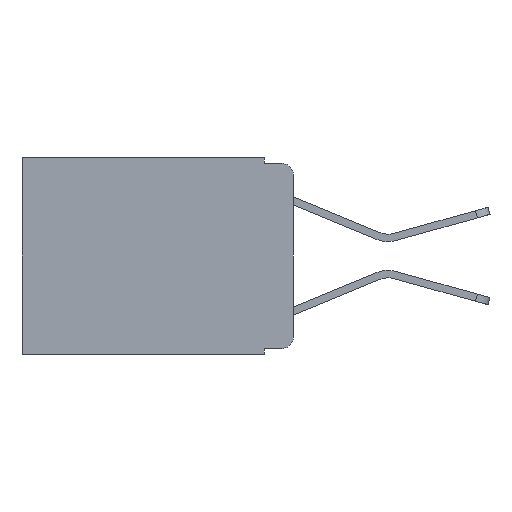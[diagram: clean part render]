
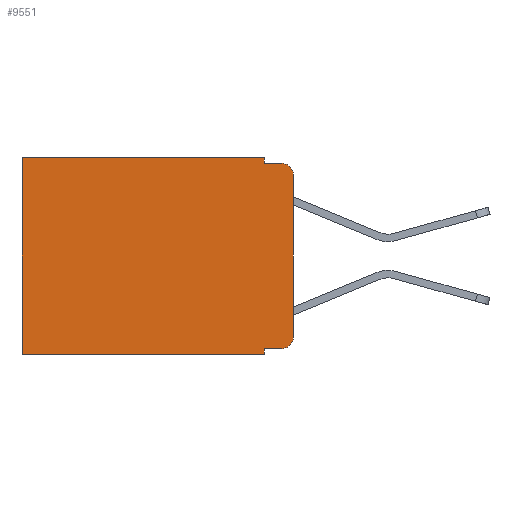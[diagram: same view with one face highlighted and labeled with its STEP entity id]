
A CAD part, left-side view. The second image highlights one B-rep face of the part: STEP entity #9551.
In plain terms, the highlighted planar face has unit normal (-1, 0, 0).
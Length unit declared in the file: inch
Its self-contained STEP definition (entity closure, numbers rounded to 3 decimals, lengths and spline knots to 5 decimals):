
#35 = ORIENTED_EDGE ( 'NONE', *, *, #2153, .T. ) ;
#64 = VERTEX_POINT ( 'NONE', #6441 ) ;
#159 = DIRECTION ( 'NONE',  ( 1., 0., 0. ) ) ;
#542 = ORIENTED_EDGE ( 'NONE', *, *, #681, .F. ) ;
#681 = EDGE_CURVE ( 'NONE', #5882, #8340, #4499, .T. ) ;
#957 = LINE ( 'NONE', #4691, #6111 ) ;
#1182 = ORIENTED_EDGE ( 'NONE', *, *, #2798, .F. ) ;
#1262 = PLANE ( 'NONE',  #4870 ) ;
#1635 = VERTEX_POINT ( 'NONE', #9061 ) ;
#1776 = CARTESIAN_POINT ( 'NONE',  ( 0.298, 0.02, -0.333 ) ) ;
#1806 = VERTEX_POINT ( 'NONE', #1776 ) ;
#2031 = EDGE_CURVE ( 'NONE', #7114, #64, #3265, .T. ) ;
#2047 = CARTESIAN_POINT ( 'NONE',  ( 0.298, 0., 0. ) ) ;
#2103 = ORIENTED_EDGE ( 'NONE', *, *, #3452, .F. ) ;
#2153 = EDGE_CURVE ( 'NONE', #5882, #10709, #8374, .T. ) ;
#2289 = CARTESIAN_POINT ( 'NONE',  ( 0.298, 0.051, -0.01 ) ) ;
#2487 = DIRECTION ( 'NONE',  ( 0., 0., -1. ) ) ;
#2606 = VECTOR ( 'NONE', #7270, 39.37008 ) ;
#2651 = ORIENTED_EDGE ( 'NONE', *, *, #5917, .T. ) ;
#2798 = EDGE_CURVE ( 'NONE', #9200, #10709, #957, .T. ) ;
#2937 = VECTOR ( 'NONE', #7928, 39.37008 ) ;
#3265 = LINE ( 'NONE', #3336, #10334 ) ;
#3299 = ORIENTED_EDGE ( 'NONE', *, *, #4711, .F. ) ;
#3336 = CARTESIAN_POINT ( 'NONE',  ( 0.298, 0., 0. ) ) ;
#3452 = EDGE_CURVE ( 'NONE', #7114, #9200, #7149, .T. ) ;
#4063 = VECTOR ( 'NONE', #5089, 39.37008 ) ;
#4067 = CARTESIAN_POINT ( 'NONE',  ( 0.298, 0.02, -0.313 ) ) ;
#4089 = EDGE_CURVE ( 'NONE', #64, #11392, #5932, .T. ) ;
#4499 = LINE ( 'NONE', #2047, #6854 ) ;
#4644 = ORIENTED_EDGE ( 'NONE', *, *, #4089, .T. ) ;
#4691 = CARTESIAN_POINT ( 'NONE',  ( 0.298, 0.051, -0.01 ) ) ;
#4711 = EDGE_CURVE ( 'NONE', #8566, #1635, #8681, .T. ) ;
#4870 = AXIS2_PLACEMENT_3D ( 'NONE', #6087, #159, #6940 ) ;
#4994 = DIRECTION ( 'NONE',  ( 0., 0., -1. ) ) ;
#5055 = VECTOR ( 'NONE', #8548, 39.37008 ) ;
#5089 = DIRECTION ( 'NONE',  ( 0., 0., -1. ) ) ;
#5158 = CARTESIAN_POINT ( 'NONE',  ( 0.298, 0., -0.313 ) ) ;
#5197 = CARTESIAN_POINT ( 'NONE',  ( 0.298, 0.051, 0. ) ) ;
#5329 = EDGE_CURVE ( 'NONE', #8566, #1806, #11575, .T. ) ;
#5657 = VECTOR ( 'NONE', #9288, 39.37008 ) ;
#5766 = ORIENTED_EDGE ( 'NONE', *, *, #2031, .T. ) ;
#5817 = CARTESIAN_POINT ( 'NONE',  ( 0.298, 0., -0.03 ) ) ;
#5882 = VERTEX_POINT ( 'NONE', #5817 ) ;
#5917 = EDGE_CURVE ( 'NONE', #1806, #8340, #8536, .T. ) ;
#5932 = LINE ( 'NONE', #9080, #5657 ) ;
#5950 = DIRECTION ( 'NONE',  ( -1., 0., 0. ) ) ;
#6087 = CARTESIAN_POINT ( 'NONE',  ( 0.298, 0., 0. ) ) ;
#6095 = AXIS2_PLACEMENT_3D ( 'NONE', #8267, #5950, #7461 ) ;
#6111 = VECTOR ( 'NONE', #7453, 39.37008 ) ;
#6174 = EDGE_LOOP ( 'NONE', ( #542, #35, #1182, #2103, #5766, #4644, #7243, #3299, #9408, #2651 ) ) ;
#6441 = CARTESIAN_POINT ( 'NONE',  ( 0.298, 0.473, 0. ) ) ;
#6652 = CARTESIAN_POINT ( 'NONE',  ( 0.298, 0.051, 0. ) ) ;
#6854 = VECTOR ( 'NONE', #2487, 39.37008 ) ;
#6940 = DIRECTION ( 'NONE',  ( 0., 0., -1. ) ) ;
#7114 = VERTEX_POINT ( 'NONE', #9785 ) ;
#7149 = LINE ( 'NONE', #6652, #2606 ) ;
#7243 = ORIENTED_EDGE ( 'NONE', *, *, #10628, .F. ) ;
#7270 = DIRECTION ( 'NONE',  ( 0., 0., -1. ) ) ;
#7453 = DIRECTION ( 'NONE',  ( 0., -1., 0. ) ) ;
#7461 = DIRECTION ( 'NONE',  ( 0., 0., -1. ) ) ;
#7880 = CARTESIAN_POINT ( 'NONE',  ( 0.298, 0.473, -0.343 ) ) ;
#7928 = DIRECTION ( 'NONE',  ( 0., 1., 0. ) ) ;
#8036 = CARTESIAN_POINT ( 'NONE',  ( 0.298, 0.02, -0.01 ) ) ;
#8267 = CARTESIAN_POINT ( 'NONE',  ( 0.298, 0.02, -0.03 ) ) ;
#8340 = VERTEX_POINT ( 'NONE', #5158 ) ;
#8374 = CIRCLE ( 'NONE', #6095, 0.02 ) ;
#8383 = DIRECTION ( 'NONE',  ( 0., 1., 0. ) ) ;
#8536 = CIRCLE ( 'NONE', #10679, 0.02 ) ;
#8548 = DIRECTION ( 'NONE',  ( 0., -1., 0. ) ) ;
#8566 = VERTEX_POINT ( 'NONE', #10351 ) ;
#8681 = LINE ( 'NONE', #5197, #4063 ) ;
#8850 = CARTESIAN_POINT ( 'NONE',  ( 0.298, 0.051, -0.333 ) ) ;
#9000 = FACE_OUTER_BOUND ( 'NONE', #6174, .T. ) ;
#9061 = CARTESIAN_POINT ( 'NONE',  ( 0.298, 0.051, -0.343 ) ) ;
#9080 = CARTESIAN_POINT ( 'NONE',  ( 0.298, 0.473, 0. ) ) ;
#9200 = VERTEX_POINT ( 'NONE', #2289 ) ;
#9288 = DIRECTION ( 'NONE',  ( 0., 0., -1. ) ) ;
#9351 = LINE ( 'NONE', #11084, #2937 ) ;
#9408 = ORIENTED_EDGE ( 'NONE', *, *, #5329, .T. ) ;
#9551 = ADVANCED_FACE ( 'NONE', ( #9000 ), #1262, .F. ) ;
#9785 = CARTESIAN_POINT ( 'NONE',  ( 0.298, 0.051, 0. ) ) ;
#9980 = DIRECTION ( 'NONE',  ( -1., 0., 0. ) ) ;
#10334 = VECTOR ( 'NONE', #8383, 39.37008 ) ;
#10351 = CARTESIAN_POINT ( 'NONE',  ( 0.298, 0.051, -0.333 ) ) ;
#10628 = EDGE_CURVE ( 'NONE', #1635, #11392, #9351, .T. ) ;
#10679 = AXIS2_PLACEMENT_3D ( 'NONE', #4067, #9980, #4994 ) ;
#10709 = VERTEX_POINT ( 'NONE', #8036 ) ;
#11084 = CARTESIAN_POINT ( 'NONE',  ( 0.298, 0., -0.343 ) ) ;
#11392 = VERTEX_POINT ( 'NONE', #7880 ) ;
#11575 = LINE ( 'NONE', #8850, #5055 ) ;
